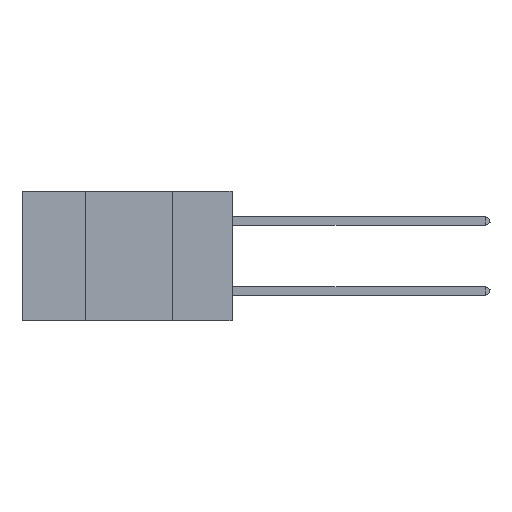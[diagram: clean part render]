
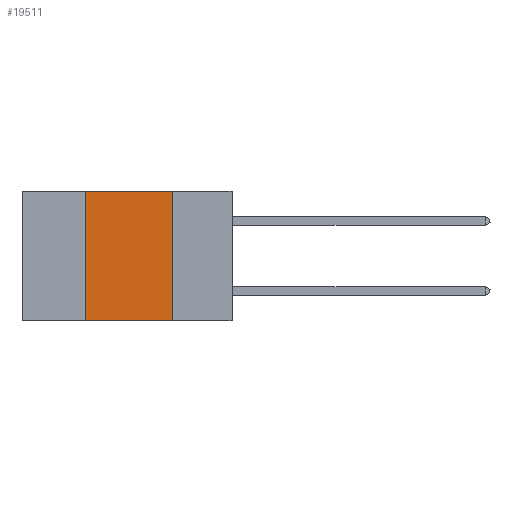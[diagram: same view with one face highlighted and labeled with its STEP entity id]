
A CAD part, left-side view. The second image highlights one B-rep face of the part: STEP entity #19511.
In plain terms, the highlighted planar face has unit normal (-1, 0, 0).
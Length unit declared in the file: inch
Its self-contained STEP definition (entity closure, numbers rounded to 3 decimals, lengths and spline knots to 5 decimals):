
#70 = ORIENTED_EDGE ( 'NONE', *, *, #36112, .F. ) ;
#192 = VERTEX_POINT ( 'NONE', #31371 ) ;
#2348 = VECTOR ( 'NONE', #46439, 39.37008 ) ;
#4030 = FACE_OUTER_BOUND ( 'NONE', #28181, .T. ) ;
#5026 = EDGE_CURVE ( 'NONE', #13209, #192, #23963, .T. ) ;
#6794 = CARTESIAN_POINT ( 'NONE',  ( 0., 0.42, 0. ) ) ;
#9140 = VECTOR ( 'NONE', #38247, 39.37008 ) ;
#10745 = CARTESIAN_POINT ( 'NONE',  ( 0., 0.42, -0.37 ) ) ;
#10804 = AXIS2_PLACEMENT_3D ( 'NONE', #21971, #33016, #29436 ) ;
#12146 = CARTESIAN_POINT ( 'NONE',  ( 0., 0.6, 0. ) ) ;
#12960 = CARTESIAN_POINT ( 'NONE',  ( 0., 0.6, -0.37 ) ) ;
#13209 = VERTEX_POINT ( 'NONE', #10745 ) ;
#13442 = VECTOR ( 'NONE', #46131, 39.37008 ) ;
#14820 = VERTEX_POINT ( 'NONE', #34216 ) ;
#17728 = EDGE_CURVE ( 'NONE', #13209, #14820, #23656, .T. ) ;
#19511 = ADVANCED_FACE ( 'NONE', ( #4030 ), #25696, .F. ) ;
#21971 = CARTESIAN_POINT ( 'NONE',  ( 0., 0.6, 0. ) ) ;
#23656 = LINE ( 'NONE', #12960, #2348 ) ;
#23853 = CARTESIAN_POINT ( 'NONE',  ( 0., 0.17, 0. ) ) ;
#23963 = LINE ( 'NONE', #6794, #34999 ) ;
#23991 = CARTESIAN_POINT ( 'NONE',  ( 0., 0.17, 0. ) ) ;
#25696 = PLANE ( 'NONE',  #10804 ) ;
#28181 = EDGE_LOOP ( 'NONE', ( #70, #33231, #31452, #45841 ) ) ;
#29436 = DIRECTION ( 'NONE',  ( 0., 0., -1. ) ) ;
#29642 = EDGE_CURVE ( 'NONE', #192, #41522, #47611, .T. ) ;
#31371 = CARTESIAN_POINT ( 'NONE',  ( 0., 0.42, 0. ) ) ;
#31452 = ORIENTED_EDGE ( 'NONE', *, *, #5026, .F. ) ;
#33016 = DIRECTION ( 'NONE',  ( 1., 0., 0. ) ) ;
#33062 = DIRECTION ( 'NONE',  ( 0., 0., 1. ) ) ;
#33231 = ORIENTED_EDGE ( 'NONE', *, *, #29642, .F. ) ;
#34216 = CARTESIAN_POINT ( 'NONE',  ( 0., 0.17, -0.37 ) ) ;
#34999 = VECTOR ( 'NONE', #33062, 39.37008 ) ;
#36112 = EDGE_CURVE ( 'NONE', #41522, #14820, #41937, .T. ) ;
#38247 = DIRECTION ( 'NONE',  ( 0., -1., 0. ) ) ;
#41522 = VERTEX_POINT ( 'NONE', #23853 ) ;
#41937 = LINE ( 'NONE', #23991, #13442 ) ;
#45841 = ORIENTED_EDGE ( 'NONE', *, *, #17728, .T. ) ;
#46131 = DIRECTION ( 'NONE',  ( 0., 0., -1. ) ) ;
#46439 = DIRECTION ( 'NONE',  ( 0., -1., 0. ) ) ;
#47611 = LINE ( 'NONE', #12146, #9140 ) ;
